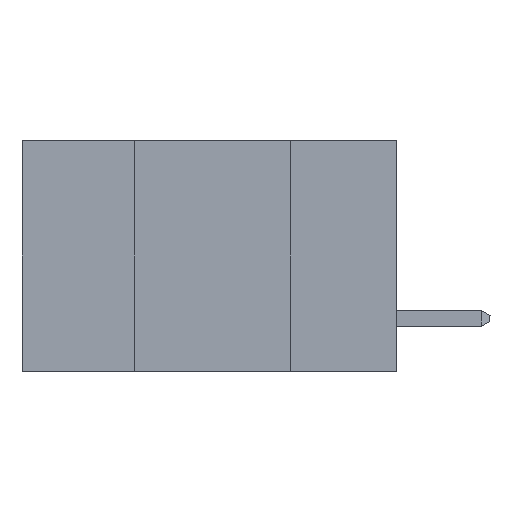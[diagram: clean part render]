
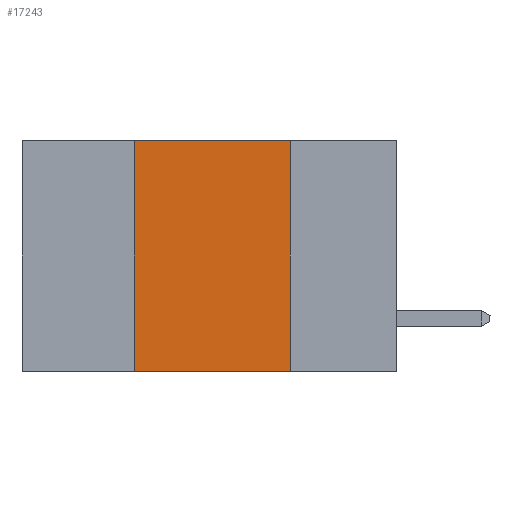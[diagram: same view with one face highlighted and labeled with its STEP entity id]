
A CAD part, left-side view. The second image highlights one B-rep face of the part: STEP entity #17243.
In plain terms, the highlighted planar face has unit normal (-1, 0, 0).
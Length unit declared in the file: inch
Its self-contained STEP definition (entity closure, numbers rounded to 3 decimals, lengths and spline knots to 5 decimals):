
#513 = VECTOR ( 'NONE', #8023, 39.37008 ) ;
#571 = EDGE_CURVE ( 'NONE', #15079, #2318, #18147, .T. ) ;
#901 = DIRECTION ( 'NONE',  ( 0., -1., 0. ) ) ;
#2318 = VERTEX_POINT ( 'NONE', #23011 ) ;
#2350 = CARTESIAN_POINT ( 'NONE',  ( 0., 0.17, 0. ) ) ;
#2520 = AXIS2_PLACEMENT_3D ( 'NONE', #15470, #20059, #22438 ) ;
#6535 = DIRECTION ( 'NONE',  ( 0., -1., 0. ) ) ;
#8023 = DIRECTION ( 'NONE',  ( 0., 0., 1. ) ) ;
#9467 = ORIENTED_EDGE ( 'NONE', *, *, #571, .T. ) ;
#12677 = LINE ( 'NONE', #17099, #513 ) ;
#13658 = CARTESIAN_POINT ( 'NONE',  ( 0., 0.42, -0.37 ) ) ;
#14594 = CARTESIAN_POINT ( 'NONE',  ( 0., 0.6, 0. ) ) ;
#14634 = EDGE_CURVE ( 'NONE', #21124, #22009, #23799, .T. ) ;
#15079 = VERTEX_POINT ( 'NONE', #13658 ) ;
#15295 = VECTOR ( 'NONE', #22666, 39.37008 ) ;
#15470 = CARTESIAN_POINT ( 'NONE',  ( 0., 0.6, 0. ) ) ;
#15767 = ORIENTED_EDGE ( 'NONE', *, *, #27864, .F. ) ;
#15866 = EDGE_CURVE ( 'NONE', #15079, #21124, #12677, .T. ) ;
#17099 = CARTESIAN_POINT ( 'NONE',  ( 0., 0.42, 0. ) ) ;
#17243 = ADVANCED_FACE ( 'NONE', ( #20084 ), #29090, .F. ) ;
#17730 = VECTOR ( 'NONE', #901, 39.37008 ) ;
#17870 = CARTESIAN_POINT ( 'NONE',  ( 0., 0.42, 0. ) ) ;
#17981 = EDGE_LOOP ( 'NONE', ( #15767, #24420, #19555, #9467 ) ) ;
#18147 = LINE ( 'NONE', #29522, #25983 ) ;
#19555 = ORIENTED_EDGE ( 'NONE', *, *, #15866, .F. ) ;
#20059 = DIRECTION ( 'NONE',  ( 1., 0., 0. ) ) ;
#20084 = FACE_OUTER_BOUND ( 'NONE', #17981, .T. ) ;
#20305 = LINE ( 'NONE', #29219, #15295 ) ;
#21124 = VERTEX_POINT ( 'NONE', #17870 ) ;
#22009 = VERTEX_POINT ( 'NONE', #2350 ) ;
#22438 = DIRECTION ( 'NONE',  ( 0., 0., -1. ) ) ;
#22666 = DIRECTION ( 'NONE',  ( 0., 0., -1. ) ) ;
#23011 = CARTESIAN_POINT ( 'NONE',  ( 0., 0.17, -0.37 ) ) ;
#23799 = LINE ( 'NONE', #14594, #17730 ) ;
#24420 = ORIENTED_EDGE ( 'NONE', *, *, #14634, .F. ) ;
#25983 = VECTOR ( 'NONE', #6535, 39.37008 ) ;
#27864 = EDGE_CURVE ( 'NONE', #22009, #2318, #20305, .T. ) ;
#29090 = PLANE ( 'NONE',  #2520 ) ;
#29219 = CARTESIAN_POINT ( 'NONE',  ( 0., 0.17, 0. ) ) ;
#29522 = CARTESIAN_POINT ( 'NONE',  ( 0., 0.6, -0.37 ) ) ;
